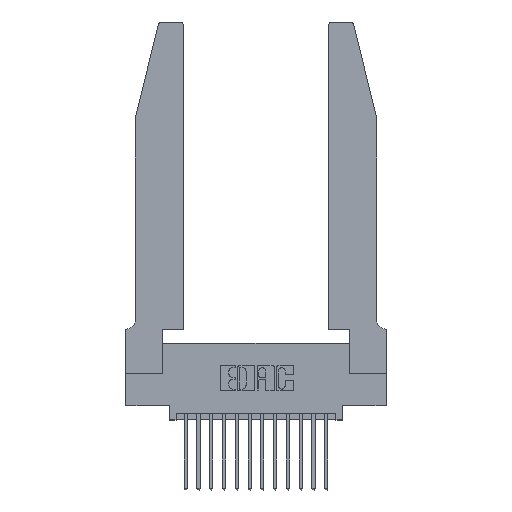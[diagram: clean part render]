
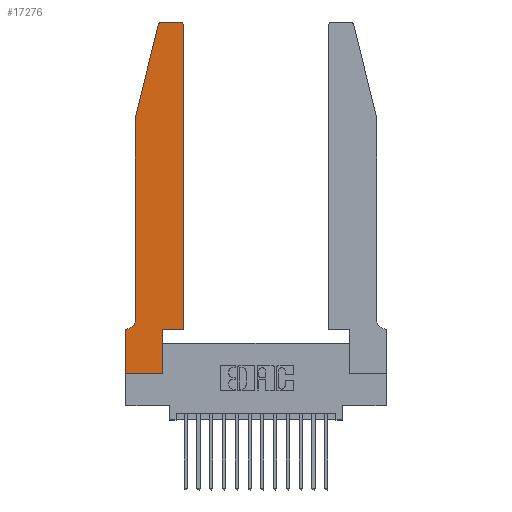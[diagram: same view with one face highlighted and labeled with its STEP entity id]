
A CAD part, top view. The second image highlights one B-rep face of the part: STEP entity #17276.
In plain terms, the highlighted planar face has unit normal (0, 0, 1).
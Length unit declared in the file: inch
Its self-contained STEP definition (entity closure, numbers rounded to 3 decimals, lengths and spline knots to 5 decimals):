
#34 = ORIENTED_EDGE ( 'NONE', *, *, #4352, .T. ) ;
#314 = LINE ( 'NONE', #12830, #18304 ) ;
#576 = AXIS2_PLACEMENT_3D ( 'NONE', #4872, #3275, #4263 ) ;
#611 = PLANE ( 'NONE',  #16624 ) ;
#1043 = ORIENTED_EDGE ( 'NONE', *, *, #10881, .T. ) ;
#1294 = LINE ( 'NONE', #10479, #12365 ) ;
#1393 = VECTOR ( 'NONE', #18346, 39.37008 ) ;
#1553 = ORIENTED_EDGE ( 'NONE', *, *, #7502, .T. ) ;
#1610 = EDGE_CURVE ( 'NONE', #6512, #5124, #9229, .T. ) ;
#1774 = DIRECTION ( 'NONE',  ( -1., 0., 0. ) ) ;
#2019 = LINE ( 'NONE', #11596, #9320 ) ;
#2067 = ORIENTED_EDGE ( 'NONE', *, *, #17749, .T. ) ;
#2172 = DIRECTION ( 'NONE',  ( 1., 0., 0. ) ) ;
#2390 = DIRECTION ( 'NONE',  ( 1., 0., 0. ) ) ;
#2435 = EDGE_CURVE ( 'NONE', #5124, #11526, #314, .T. ) ;
#2573 = LINE ( 'NONE', #8609, #17221 ) ;
#2693 = FACE_OUTER_BOUND ( 'NONE', #6627, .T. ) ;
#2817 = ORIENTED_EDGE ( 'NONE', *, *, #9581, .T. ) ;
#2819 = DIRECTION ( 'NONE',  ( -1., 0., 0. ) ) ;
#3240 = CIRCLE ( 'NONE', #576, 0.03 ) ;
#3266 = DIRECTION ( 'NONE',  ( 0., -1., 0. ) ) ;
#3274 = VERTEX_POINT ( 'NONE', #13534 ) ;
#3275 = DIRECTION ( 'NONE',  ( 0., 0., 1. ) ) ;
#3290 = CARTESIAN_POINT ( 'NONE',  ( 0.4205, 2.72, 0.37 ) ) ;
#3323 = EDGE_CURVE ( 'NONE', #7024, #6512, #2573, .T. ) ;
#3727 = VECTOR ( 'NONE', #7922, 39.37008 ) ;
#3734 = VERTEX_POINT ( 'NONE', #10710 ) ;
#3783 = LINE ( 'NONE', #16580, #11412 ) ;
#3936 = EDGE_CURVE ( 'NONE', #14317, #8117, #8682, .T. ) ;
#4263 = DIRECTION ( 'NONE',  ( 1., 0., 0. ) ) ;
#4273 = EDGE_CURVE ( 'NONE', #13971, #3734, #15039, .T. ) ;
#4302 = DIRECTION ( 'NONE',  ( -0.239, -0.971, 0. ) ) ;
#4352 = EDGE_CURVE ( 'NONE', #9319, #6408, #3240, .T. ) ;
#4520 = AXIS2_PLACEMENT_3D ( 'NONE', #3290, #13289, #4767 ) ;
#4767 = DIRECTION ( 'NONE',  ( 1., 0., 0. ) ) ;
#4872 = CARTESIAN_POINT ( 'NONE',  ( 0.284, 2.72, 0.37 ) ) ;
#5041 = DIRECTION ( 'NONE',  ( 1., 0., 0. ) ) ;
#5124 = VERTEX_POINT ( 'NONE', #14417 ) ;
#5136 = CARTESIAN_POINT ( 'NONE',  ( 0.4505, 0.35, 0.37 ) ) ;
#5207 = VECTOR ( 'NONE', #4302, 39.37008 ) ;
#5789 = ORIENTED_EDGE ( 'NONE', *, *, #6338, .T. ) ;
#5793 = LINE ( 'NONE', #5136, #9180 ) ;
#5904 = CARTESIAN_POINT ( 'NONE',  ( 0.4505, 2.72, 0.37 ) ) ;
#6151 = ORIENTED_EDGE ( 'NONE', *, *, #15143, .T. ) ;
#6338 = EDGE_CURVE ( 'NONE', #11526, #18059, #2019, .T. ) ;
#6408 = VERTEX_POINT ( 'NONE', #11713 ) ;
#6423 = CARTESIAN_POINT ( 'NONE',  ( 0., 0.35, 0.37 ) ) ;
#6512 = VERTEX_POINT ( 'NONE', #10532 ) ;
#6627 = EDGE_LOOP ( 'NONE', ( #2067, #34, #1553, #11547, #9136, #18250, #5789, #2817, #13633, #1043, #17507, #6151 ) ) ;
#7024 = VERTEX_POINT ( 'NONE', #15805 ) ;
#7337 = DIRECTION ( 'NONE',  ( 0., -1., 0. ) ) ;
#7502 = EDGE_CURVE ( 'NONE', #6408, #7024, #16902, .T. ) ;
#7689 = CARTESIAN_POINT ( 'NONE',  ( 0.2865, 0., 0.37 ) ) ;
#7922 = DIRECTION ( 'NONE',  ( 0., 1., 0. ) ) ;
#8117 = VERTEX_POINT ( 'NONE', #5904 ) ;
#8566 = CARTESIAN_POINT ( 'NONE',  ( 0.0755, 2., 0.37 ) ) ;
#8609 = CARTESIAN_POINT ( 'NONE',  ( 0.0755, 2., 0.37 ) ) ;
#8682 = LINE ( 'NONE', #10445, #1393 ) ;
#9016 = CARTESIAN_POINT ( 'NONE',  ( 0.284, 2.75, 0.37 ) ) ;
#9136 = ORIENTED_EDGE ( 'NONE', *, *, #1610, .T. ) ;
#9180 = VECTOR ( 'NONE', #2172, 39.37008 ) ;
#9229 = CIRCLE ( 'NONE', #16141, 0.07 ) ;
#9319 = VERTEX_POINT ( 'NONE', #9016 ) ;
#9320 = VECTOR ( 'NONE', #7337, 39.37008 ) ;
#9349 = CARTESIAN_POINT ( 'NONE',  ( 0., 0.35, 0.37 ) ) ;
#9581 = EDGE_CURVE ( 'NONE', #18059, #13971, #3783, .T. ) ;
#10102 = CARTESIAN_POINT ( 'NONE',  ( 0.0055, 0.42, 0.37 ) ) ;
#10445 = CARTESIAN_POINT ( 'NONE',  ( 0.4505, 0.35, 0.37 ) ) ;
#10479 = CARTESIAN_POINT ( 'NONE',  ( 0.2605, 2.75, 0.37 ) ) ;
#10532 = CARTESIAN_POINT ( 'NONE',  ( 0.0755, 0.42, 0.37 ) ) ;
#10578 = DIRECTION ( 'NONE',  ( 0., 0., -1. ) ) ;
#10610 = CIRCLE ( 'NONE', #4520, 0.03 ) ;
#10710 = CARTESIAN_POINT ( 'NONE',  ( 0.2865, 0.35, 0.37 ) ) ;
#10881 = EDGE_CURVE ( 'NONE', #3734, #14317, #5793, .T. ) ;
#11412 = VECTOR ( 'NONE', #2390, 39.37008 ) ;
#11526 = VERTEX_POINT ( 'NONE', #9349 ) ;
#11547 = ORIENTED_EDGE ( 'NONE', *, *, #3323, .T. ) ;
#11596 = CARTESIAN_POINT ( 'NONE',  ( 0., 0., 0.37 ) ) ;
#11713 = CARTESIAN_POINT ( 'NONE',  ( 0.25487, 2.72718, 0.37 ) ) ;
#12365 = VECTOR ( 'NONE', #1774, 39.37008 ) ;
#12830 = CARTESIAN_POINT ( 'NONE',  ( 0.0755, 0.35, 0.37 ) ) ;
#13289 = DIRECTION ( 'NONE',  ( 0., 0., 1. ) ) ;
#13534 = CARTESIAN_POINT ( 'NONE',  ( 0.4205, 2.75, 0.37 ) ) ;
#13554 = DIRECTION ( 'NONE',  ( 0., 0., 1. ) ) ;
#13633 = ORIENTED_EDGE ( 'NONE', *, *, #4273, .T. ) ;
#13971 = VERTEX_POINT ( 'NONE', #7689 ) ;
#14121 = CARTESIAN_POINT ( 'NONE',  ( 0., 0., 0.37 ) ) ;
#14317 = VERTEX_POINT ( 'NONE', #18123 ) ;
#14417 = CARTESIAN_POINT ( 'NONE',  ( 0.0055, 0.35, 0.37 ) ) ;
#14469 = DIRECTION ( 'NONE',  ( -1., 0., 0. ) ) ;
#15039 = LINE ( 'NONE', #15232, #3727 ) ;
#15143 = EDGE_CURVE ( 'NONE', #8117, #3274, #10610, .T. ) ;
#15232 = CARTESIAN_POINT ( 'NONE',  ( 0.2865, 0.35, 0.37 ) ) ;
#15805 = CARTESIAN_POINT ( 'NONE',  ( 0.0755, 2., 0.37 ) ) ;
#16141 = AXIS2_PLACEMENT_3D ( 'NONE', #10102, #10578, #14469 ) ;
#16580 = CARTESIAN_POINT ( 'NONE',  ( 0., 0., 0.37 ) ) ;
#16624 = AXIS2_PLACEMENT_3D ( 'NONE', #6423, #13554, #5041 ) ;
#16902 = LINE ( 'NONE', #8566, #5207 ) ;
#17221 = VECTOR ( 'NONE', #3266, 39.37008 ) ;
#17276 = ADVANCED_FACE ( 'NONE', ( #2693 ), #611, .T. ) ;
#17507 = ORIENTED_EDGE ( 'NONE', *, *, #3936, .T. ) ;
#17749 = EDGE_CURVE ( 'NONE', #3274, #9319, #1294, .T. ) ;
#18059 = VERTEX_POINT ( 'NONE', #14121 ) ;
#18123 = CARTESIAN_POINT ( 'NONE',  ( 0.4505, 0.35, 0.37 ) ) ;
#18250 = ORIENTED_EDGE ( 'NONE', *, *, #2435, .T. ) ;
#18304 = VECTOR ( 'NONE', #2819, 39.37008 ) ;
#18346 = DIRECTION ( 'NONE',  ( 0., 1., 0. ) ) ;
